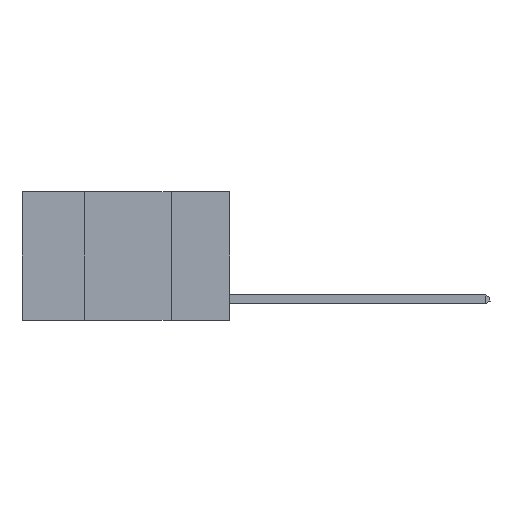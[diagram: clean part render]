
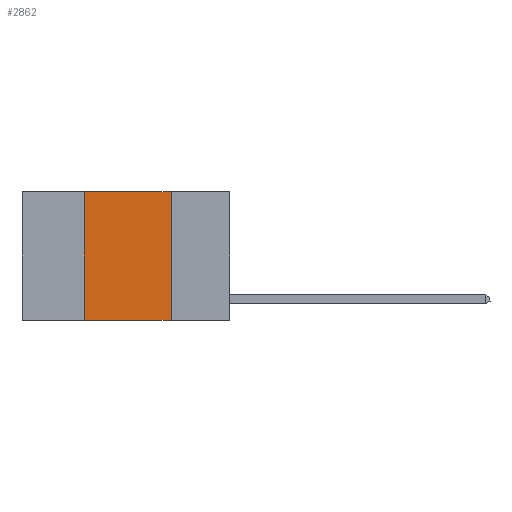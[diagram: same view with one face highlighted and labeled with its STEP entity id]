
A CAD part, left-side view. The second image highlights one B-rep face of the part: STEP entity #2862.
In plain terms, the highlighted planar face has unit normal (-1, 0, 0).
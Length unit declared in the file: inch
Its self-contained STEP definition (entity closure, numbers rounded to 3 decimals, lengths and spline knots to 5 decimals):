
#354 = LINE ( 'NONE', #3128, #10195 ) ;
#654 = EDGE_CURVE ( 'NONE', #15197, #8317, #4806, .T. ) ;
#790 = VECTOR ( 'NONE', #14105, 39.37008 ) ;
#1087 = DIRECTION ( 'NONE',  ( 0., 0., -1. ) ) ;
#1912 = VERTEX_POINT ( 'NONE', #15992 ) ;
#2185 = DIRECTION ( 'NONE',  ( 1., 0., 0. ) ) ;
#2862 = ADVANCED_FACE ( 'NONE', ( #6033 ), #5179, .F. ) ;
#3128 = CARTESIAN_POINT ( 'NONE',  ( 0., 0.6, -0.37 ) ) ;
#3304 = LINE ( 'NONE', #9669, #790 ) ;
#4293 = ORIENTED_EDGE ( 'NONE', *, *, #6335, .F. ) ;
#4389 = VECTOR ( 'NONE', #1087, 39.37008 ) ;
#4806 = LINE ( 'NONE', #7530, #4389 ) ;
#5179 = PLANE ( 'NONE',  #11892 ) ;
#6033 = FACE_OUTER_BOUND ( 'NONE', #15820, .T. ) ;
#6335 = EDGE_CURVE ( 'NONE', #9406, #1912, #11785, .T. ) ;
#7386 = CARTESIAN_POINT ( 'NONE',  ( 0., 0.6, 0. ) ) ;
#7499 = ORIENTED_EDGE ( 'NONE', *, *, #654, .F. ) ;
#7530 = CARTESIAN_POINT ( 'NONE',  ( 0., 0.17, 0. ) ) ;
#8317 = VERTEX_POINT ( 'NONE', #15127 ) ;
#9406 = VERTEX_POINT ( 'NONE', #15095 ) ;
#9502 = ORIENTED_EDGE ( 'NONE', *, *, #15926, .F. ) ;
#9669 = CARTESIAN_POINT ( 'NONE',  ( 0., 0.6, 0. ) ) ;
#10047 = DIRECTION ( 'NONE',  ( 0., 0., 1. ) ) ;
#10195 = VECTOR ( 'NONE', #15251, 39.37008 ) ;
#10245 = ORIENTED_EDGE ( 'NONE', *, *, #10783, .T. ) ;
#10783 = EDGE_CURVE ( 'NONE', #9406, #8317, #354, .T. ) ;
#11785 = LINE ( 'NONE', #16797, #16435 ) ;
#11892 = AXIS2_PLACEMENT_3D ( 'NONE', #7386, #2185, #14198 ) ;
#13081 = CARTESIAN_POINT ( 'NONE',  ( 0., 0.17, 0. ) ) ;
#14105 = DIRECTION ( 'NONE',  ( 0., -1., 0. ) ) ;
#14198 = DIRECTION ( 'NONE',  ( 0., 0., -1. ) ) ;
#15095 = CARTESIAN_POINT ( 'NONE',  ( 0., 0.42, -0.37 ) ) ;
#15127 = CARTESIAN_POINT ( 'NONE',  ( 0., 0.17, -0.37 ) ) ;
#15197 = VERTEX_POINT ( 'NONE', #13081 ) ;
#15251 = DIRECTION ( 'NONE',  ( 0., -1., 0. ) ) ;
#15820 = EDGE_LOOP ( 'NONE', ( #7499, #9502, #4293, #10245 ) ) ;
#15926 = EDGE_CURVE ( 'NONE', #1912, #15197, #3304, .T. ) ;
#15992 = CARTESIAN_POINT ( 'NONE',  ( 0., 0.42, 0. ) ) ;
#16435 = VECTOR ( 'NONE', #10047, 39.37008 ) ;
#16797 = CARTESIAN_POINT ( 'NONE',  ( 0., 0.42, 0. ) ) ;
